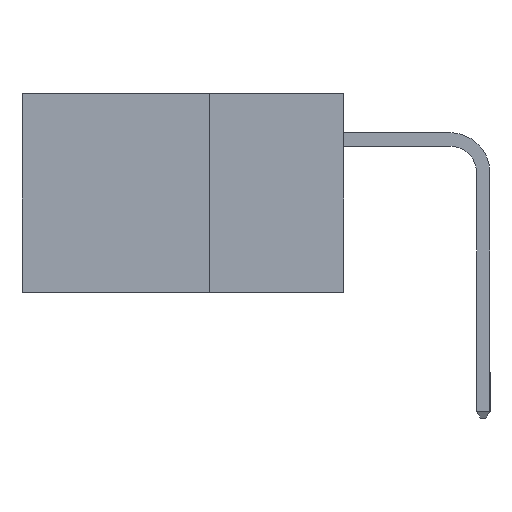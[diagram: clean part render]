
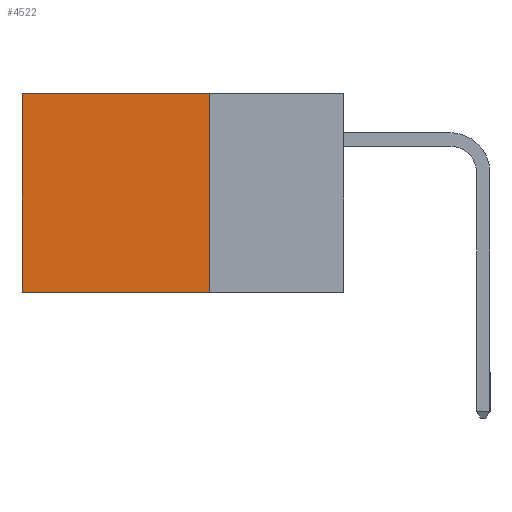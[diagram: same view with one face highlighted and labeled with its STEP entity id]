
A CAD part, left-side view. The second image highlights one B-rep face of the part: STEP entity #4522.
In plain terms, the highlighted planar face has unit normal (-1, 0, 0).
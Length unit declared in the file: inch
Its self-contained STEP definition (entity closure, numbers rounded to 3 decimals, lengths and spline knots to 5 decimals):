
#198 = ORIENTED_EDGE ( 'NONE', *, *, #10255, .T. ) ;
#668 = CARTESIAN_POINT ( 'NONE',  ( 0.298, 0.25, 0. ) ) ;
#900 = DIRECTION ( 'NONE',  ( 0., 1., 0. ) ) ;
#988 = LINE ( 'NONE', #10067, #9574 ) ;
#1109 = DIRECTION ( 'NONE',  ( 0., 0., -1. ) ) ;
#1288 = VERTEX_POINT ( 'NONE', #2307 ) ;
#1473 = CARTESIAN_POINT ( 'NONE',  ( 0.298, 0.6, 0. ) ) ;
#1677 = DIRECTION ( 'NONE',  ( 0., 1., 0. ) ) ;
#1923 = ORIENTED_EDGE ( 'NONE', *, *, #5972, .F. ) ;
#2102 = CARTESIAN_POINT ( 'NONE',  ( 0.298, 0.6, 0. ) ) ;
#2307 = CARTESIAN_POINT ( 'NONE',  ( 0.298, 0.6, -0.37 ) ) ;
#2407 = LINE ( 'NONE', #11666, #2977 ) ;
#2977 = VECTOR ( 'NONE', #900, 39.37008 ) ;
#3362 = CARTESIAN_POINT ( 'NONE',  ( 0.298, 0.25, -0.37 ) ) ;
#3399 = LINE ( 'NONE', #2102, #11415 ) ;
#3560 = DIRECTION ( 'NONE',  ( 1., 0., 0. ) ) ;
#3708 = EDGE_CURVE ( 'NONE', #9161, #7307, #9745, .T. ) ;
#4504 = ORIENTED_EDGE ( 'NONE', *, *, #4662, .F. ) ;
#4522 = ADVANCED_FACE ( 'NONE', ( #11406 ), #6280, .F. ) ;
#4615 = CARTESIAN_POINT ( 'NONE',  ( 0.298, 0.25, 0. ) ) ;
#4662 = EDGE_CURVE ( 'NONE', #9161, #8568, #988, .T. ) ;
#4903 = DIRECTION ( 'NONE',  ( 0., 0., -1. ) ) ;
#5972 = EDGE_CURVE ( 'NONE', #8568, #1288, #2407, .T. ) ;
#6280 = PLANE ( 'NONE',  #8519 ) ;
#6354 = DIRECTION ( 'NONE',  ( 0., 0., -1. ) ) ;
#7307 = VERTEX_POINT ( 'NONE', #1473 ) ;
#7869 = CARTESIAN_POINT ( 'NONE',  ( 0.298, 0.25, 0. ) ) ;
#8049 = EDGE_LOOP ( 'NONE', ( #198, #1923, #4504, #9190 ) ) ;
#8070 = VECTOR ( 'NONE', #1677, 39.37008 ) ;
#8519 = AXIS2_PLACEMENT_3D ( 'NONE', #4615, #3560, #6354 ) ;
#8568 = VERTEX_POINT ( 'NONE', #3362 ) ;
#9161 = VERTEX_POINT ( 'NONE', #668 ) ;
#9190 = ORIENTED_EDGE ( 'NONE', *, *, #3708, .T. ) ;
#9574 = VECTOR ( 'NONE', #1109, 39.37008 ) ;
#9745 = LINE ( 'NONE', #7869, #8070 ) ;
#10067 = CARTESIAN_POINT ( 'NONE',  ( 0.298, 0.25, 0. ) ) ;
#10255 = EDGE_CURVE ( 'NONE', #7307, #1288, #3399, .T. ) ;
#11406 = FACE_OUTER_BOUND ( 'NONE', #8049, .T. ) ;
#11415 = VECTOR ( 'NONE', #4903, 39.37008 ) ;
#11666 = CARTESIAN_POINT ( 'NONE',  ( 0.298, 0.25, -0.37 ) ) ;
